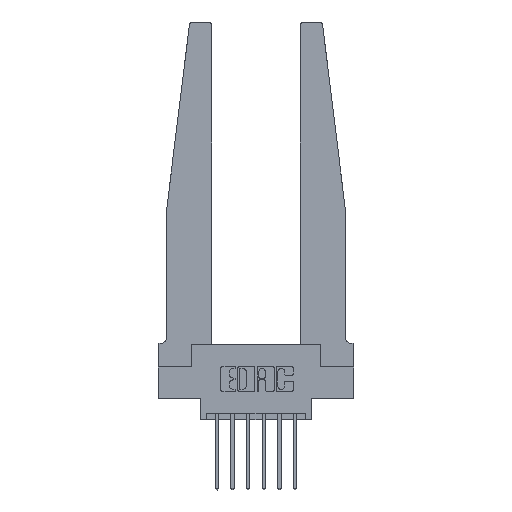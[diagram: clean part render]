
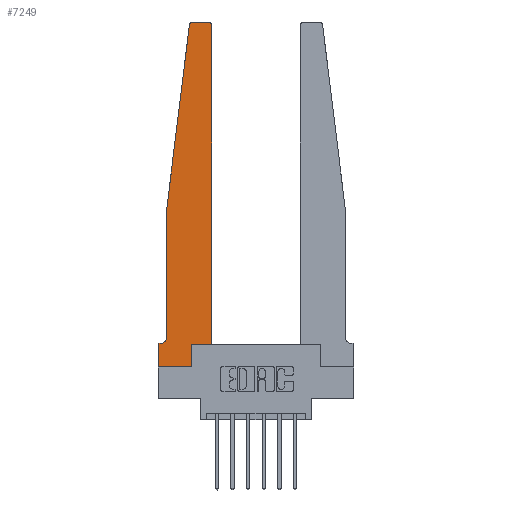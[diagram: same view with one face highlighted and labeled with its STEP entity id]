
A CAD part, top view. The second image highlights one B-rep face of the part: STEP entity #7249.
In plain terms, the highlighted planar face has unit normal (0, 0, 1).
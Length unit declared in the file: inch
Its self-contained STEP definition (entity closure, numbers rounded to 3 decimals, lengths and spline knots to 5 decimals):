
#28 = CARTESIAN_POINT ( 'NONE',  ( 0.27653, 2.72, 0.37 ) ) ;
#51 = LINE ( 'NONE', #8895, #2909 ) ;
#104 = VECTOR ( 'NONE', #13272, 39.37008 ) ;
#126 = VECTOR ( 'NONE', #10028, 39.37008 ) ;
#449 = ORIENTED_EDGE ( 'NONE', *, *, #11824, .T. ) ;
#517 = DIRECTION ( 'NONE',  ( 0., 0., 1. ) ) ;
#629 = CARTESIAN_POINT ( 'NONE',  ( 0.015, 0.2375, 0.37 ) ) ;
#863 = VERTEX_POINT ( 'NONE', #1754 ) ;
#930 = CARTESIAN_POINT ( 'NONE',  ( 0.395, 2.72, 0.37 ) ) ;
#1060 = DIRECTION ( 'NONE',  ( -1., 0., 0. ) ) ;
#1109 = DIRECTION ( 'NONE',  ( 1., 0., 0. ) ) ;
#1320 = CARTESIAN_POINT ( 'NONE',  ( 0.24675, 2.72367, 0.37 ) ) ;
#1676 = CIRCLE ( 'NONE', #2571, 0.05 ) ;
#1696 = DIRECTION ( 'NONE',  ( -1., 0., 0. ) ) ;
#1754 = CARTESIAN_POINT ( 'NONE',  ( 0.2605, 0.18, 0.37 ) ) ;
#1807 = VERTEX_POINT ( 'NONE', #5558 ) ;
#1815 = VERTEX_POINT ( 'NONE', #1320 ) ;
#1995 = DIRECTION ( 'NONE',  ( 1., 0., 0. ) ) ;
#2089 = CIRCLE ( 'NONE', #3804, 0.03 ) ;
#2498 = FACE_OUTER_BOUND ( 'NONE', #13257, .T. ) ;
#2499 = DIRECTION ( 'NONE',  ( -1., 0., 0. ) ) ;
#2571 = AXIS2_PLACEMENT_3D ( 'NONE', #629, #8056, #1696 ) ;
#2772 = ORIENTED_EDGE ( 'NONE', *, *, #2908, .T. ) ;
#2908 = EDGE_CURVE ( 'NONE', #10461, #7104, #3392, .T. ) ;
#2909 = VECTOR ( 'NONE', #2499, 39.37008 ) ;
#3070 = VECTOR ( 'NONE', #6970, 39.37008 ) ;
#3107 = LINE ( 'NONE', #7520, #8412 ) ;
#3266 = VERTEX_POINT ( 'NONE', #10694 ) ;
#3392 = LINE ( 'NONE', #11166, #3070 ) ;
#3804 = AXIS2_PLACEMENT_3D ( 'NONE', #28, #7462, #1109 ) ;
#4204 = CIRCLE ( 'NONE', #9231, 0.03 ) ;
#4226 = VECTOR ( 'NONE', #10577, 39.37008 ) ;
#4357 = ORIENTED_EDGE ( 'NONE', *, *, #9552, .T. ) ;
#4761 = PLANE ( 'NONE',  #9792 ) ;
#4848 = CARTESIAN_POINT ( 'NONE',  ( 0., 0., 0.37 ) ) ;
#5110 = LINE ( 'NONE', #13412, #5433 ) ;
#5282 = EDGE_CURVE ( 'NONE', #11271, #3266, #1676, .T. ) ;
#5433 = VECTOR ( 'NONE', #7109, 39.37008 ) ;
#5558 = CARTESIAN_POINT ( 'NONE',  ( 0.065, 1.25, 0.37 ) ) ;
#5750 = CARTESIAN_POINT ( 'NONE',  ( 0.065, 0.2375, 0.37 ) ) ;
#5863 = ORIENTED_EDGE ( 'NONE', *, *, #9495, .T. ) ;
#6358 = ORIENTED_EDGE ( 'NONE', *, *, #7395, .T. ) ;
#6462 = ORIENTED_EDGE ( 'NONE', *, *, #13208, .T. ) ;
#6485 = LINE ( 'NONE', #9253, #6803 ) ;
#6729 = CARTESIAN_POINT ( 'NONE',  ( 0.395, 2.75, 0.37 ) ) ;
#6803 = VECTOR ( 'NONE', #7119, 39.37008 ) ;
#6820 = VERTEX_POINT ( 'NONE', #12342 ) ;
#6970 = DIRECTION ( 'NONE',  ( 0., 1., 0. ) ) ;
#7104 = VERTEX_POINT ( 'NONE', #10767 ) ;
#7109 = DIRECTION ( 'NONE',  ( 0., -1., 0. ) ) ;
#7119 = DIRECTION ( 'NONE',  ( 1., 0., 0. ) ) ;
#7220 = EDGE_CURVE ( 'NONE', #863, #10461, #8478, .T. ) ;
#7249 = ADVANCED_FACE ( 'NONE', ( #2498 ), #4761, .T. ) ;
#7395 = EDGE_CURVE ( 'NONE', #12262, #6820, #6485, .T. ) ;
#7462 = DIRECTION ( 'NONE',  ( 0., 0., 1. ) ) ;
#7520 = CARTESIAN_POINT ( 'NONE',  ( 0.065, 1.25, 0.37 ) ) ;
#7736 = VERTEX_POINT ( 'NONE', #6729 ) ;
#7792 = ORIENTED_EDGE ( 'NONE', *, *, #5282, .T. ) ;
#7950 = DIRECTION ( 'NONE',  ( 1., 0., 0. ) ) ;
#8053 = LINE ( 'NONE', #9549, #10529 ) ;
#8056 = DIRECTION ( 'NONE',  ( 0., 0., -1. ) ) ;
#8196 = VERTEX_POINT ( 'NONE', #9097 ) ;
#8351 = DIRECTION ( 'NONE',  ( 0., 0., 1. ) ) ;
#8404 = ORIENTED_EDGE ( 'NONE', *, *, #12163, .T. ) ;
#8412 = VECTOR ( 'NONE', #9655, 39.37008 ) ;
#8478 = LINE ( 'NONE', #8979, #126 ) ;
#8590 = LINE ( 'NONE', #4848, #104 ) ;
#8895 = CARTESIAN_POINT ( 'NONE',  ( 0.25, 2.75, 0.37 ) ) ;
#8979 = CARTESIAN_POINT ( 'NONE',  ( 0.425, 0.18, 0.37 ) ) ;
#9097 = CARTESIAN_POINT ( 'NONE',  ( 0.27653, 2.75, 0.37 ) ) ;
#9231 = AXIS2_PLACEMENT_3D ( 'NONE', #930, #8351, #1995 ) ;
#9253 = CARTESIAN_POINT ( 'NONE',  ( 0., 0., 0.37 ) ) ;
#9495 = EDGE_CURVE ( 'NONE', #12243, #12262, #8590, .T. ) ;
#9536 = CARTESIAN_POINT ( 'NONE',  ( 0.2605, 0.18, 0.37 ) ) ;
#9549 = CARTESIAN_POINT ( 'NONE',  ( 0.065, 0.1875, 0.37 ) ) ;
#9552 = EDGE_CURVE ( 'NONE', #1807, #11271, #5110, .T. ) ;
#9655 = DIRECTION ( 'NONE',  ( -0.122, -0.992, 0. ) ) ;
#9757 = CARTESIAN_POINT ( 'NONE',  ( 0., 0.1875, 0.37 ) ) ;
#9789 = EDGE_CURVE ( 'NONE', #1815, #1807, #3107, .T. ) ;
#9792 = AXIS2_PLACEMENT_3D ( 'NONE', #12147, #517, #7950 ) ;
#9951 = CARTESIAN_POINT ( 'NONE',  ( 0.425, 0.18, 0.37 ) ) ;
#10028 = DIRECTION ( 'NONE',  ( 1., 0., 0. ) ) ;
#10275 = ORIENTED_EDGE ( 'NONE', *, *, #10308, .T. ) ;
#10307 = EDGE_CURVE ( 'NONE', #3266, #12243, #8053, .T. ) ;
#10308 = EDGE_CURVE ( 'NONE', #8196, #1815, #2089, .T. ) ;
#10461 = VERTEX_POINT ( 'NONE', #9951 ) ;
#10529 = VECTOR ( 'NONE', #1060, 39.37008 ) ;
#10577 = DIRECTION ( 'NONE',  ( 0., 1., 0. ) ) ;
#10694 = CARTESIAN_POINT ( 'NONE',  ( 0.015, 0.1875, 0.37 ) ) ;
#10767 = CARTESIAN_POINT ( 'NONE',  ( 0.425, 2.72, 0.37 ) ) ;
#10800 = CARTESIAN_POINT ( 'NONE',  ( 0., 0., 0.37 ) ) ;
#11166 = CARTESIAN_POINT ( 'NONE',  ( 0.425, 0.18, 0.37 ) ) ;
#11185 = ORIENTED_EDGE ( 'NONE', *, *, #7220, .T. ) ;
#11271 = VERTEX_POINT ( 'NONE', #5750 ) ;
#11824 = EDGE_CURVE ( 'NONE', #7736, #8196, #51, .T. ) ;
#11996 = ORIENTED_EDGE ( 'NONE', *, *, #9789, .T. ) ;
#12041 = ORIENTED_EDGE ( 'NONE', *, *, #10307, .T. ) ;
#12147 = CARTESIAN_POINT ( 'NONE',  ( 0., 0.1875, 0.37 ) ) ;
#12163 = EDGE_CURVE ( 'NONE', #6820, #863, #12641, .T. ) ;
#12243 = VERTEX_POINT ( 'NONE', #9757 ) ;
#12262 = VERTEX_POINT ( 'NONE', #10800 ) ;
#12342 = CARTESIAN_POINT ( 'NONE',  ( 0.2605, 0., 0.37 ) ) ;
#12641 = LINE ( 'NONE', #9536, #4226 ) ;
#13208 = EDGE_CURVE ( 'NONE', #7104, #7736, #4204, .T. ) ;
#13257 = EDGE_LOOP ( 'NONE', ( #449, #10275, #11996, #4357, #7792, #12041, #5863, #6358, #8404, #11185, #2772, #6462 ) ) ;
#13272 = DIRECTION ( 'NONE',  ( 0., -1., 0. ) ) ;
#13412 = CARTESIAN_POINT ( 'NONE',  ( 0.065, 1.25, 0.37 ) ) ;
